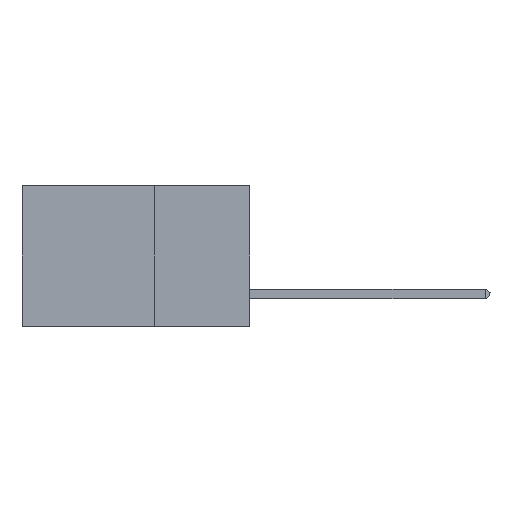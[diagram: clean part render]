
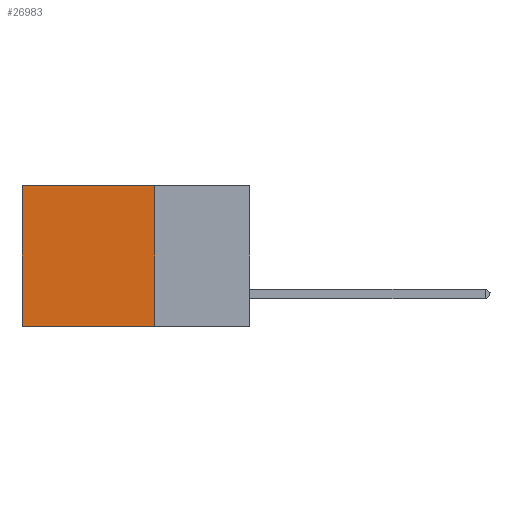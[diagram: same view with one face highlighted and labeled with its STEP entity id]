
A CAD part, left-side view. The second image highlights one B-rep face of the part: STEP entity #26983.
In plain terms, the highlighted planar face has unit normal (-1, 0, 0).
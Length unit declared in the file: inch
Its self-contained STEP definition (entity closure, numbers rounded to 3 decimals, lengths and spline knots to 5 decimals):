
#306 = VERTEX_POINT ( 'NONE', #31353 ) ;
#497 = VECTOR ( 'NONE', #8810, 39.37008 ) ;
#2908 = CARTESIAN_POINT ( 'NONE',  ( 0.2875, 0.25, 0. ) ) ;
#4172 = EDGE_CURVE ( 'NONE', #306, #19750, #36808, .T. ) ;
#5701 = CARTESIAN_POINT ( 'NONE',  ( 0.2875, 0.25, 0. ) ) ;
#5868 = PLANE ( 'NONE',  #14941 ) ;
#8810 = DIRECTION ( 'NONE',  ( 0., 1., 0. ) ) ;
#10869 = VECTOR ( 'NONE', #28611, 39.37008 ) ;
#12018 = ORIENTED_EDGE ( 'NONE', *, *, #26937, .T. ) ;
#12404 = CARTESIAN_POINT ( 'NONE',  ( 0.2875, 0.6, 0. ) ) ;
#13059 = DIRECTION ( 'NONE',  ( 1., 0., 0. ) ) ;
#13226 = CARTESIAN_POINT ( 'NONE',  ( 0.2875, 0.25, -0.37 ) ) ;
#13312 = DIRECTION ( 'NONE',  ( 0., 0., -1. ) ) ;
#13999 = FACE_OUTER_BOUND ( 'NONE', #15345, .T. ) ;
#14941 = AXIS2_PLACEMENT_3D ( 'NONE', #2908, #13059, #23271 ) ;
#15345 = EDGE_LOOP ( 'NONE', ( #32475, #23507, #39131, #12018 ) ) ;
#17144 = CARTESIAN_POINT ( 'NONE',  ( 0.2875, 0.25, 0. ) ) ;
#18142 = CARTESIAN_POINT ( 'NONE',  ( 0.2875, 0.6, -0.37 ) ) ;
#19750 = VERTEX_POINT ( 'NONE', #18142 ) ;
#20350 = VERTEX_POINT ( 'NONE', #33217 ) ;
#21724 = VECTOR ( 'NONE', #13312, 39.37008 ) ;
#22113 = LINE ( 'NONE', #5701, #497 ) ;
#22253 = LINE ( 'NONE', #17144, #24252 ) ;
#23271 = DIRECTION ( 'NONE',  ( 0., 0., -1. ) ) ;
#23507 = ORIENTED_EDGE ( 'NONE', *, *, #35232, .F. ) ;
#23815 = EDGE_CURVE ( 'NONE', #20350, #32720, #22253, .T. ) ;
#24252 = VECTOR ( 'NONE', #25397, 39.37008 ) ;
#25397 = DIRECTION ( 'NONE',  ( 0., 0., -1. ) ) ;
#26937 = EDGE_CURVE ( 'NONE', #20350, #306, #22113, .T. ) ;
#26983 = ADVANCED_FACE ( 'NONE', ( #13999 ), #5868, .F. ) ;
#27852 = CARTESIAN_POINT ( 'NONE',  ( 0.2875, 0.25, -0.37 ) ) ;
#28611 = DIRECTION ( 'NONE',  ( 0., 1., 0. ) ) ;
#31353 = CARTESIAN_POINT ( 'NONE',  ( 0.2875, 0.6, 0. ) ) ;
#32475 = ORIENTED_EDGE ( 'NONE', *, *, #4172, .T. ) ;
#32720 = VERTEX_POINT ( 'NONE', #27852 ) ;
#33217 = CARTESIAN_POINT ( 'NONE',  ( 0.2875, 0.25, 0. ) ) ;
#33302 = LINE ( 'NONE', #13226, #10869 ) ;
#35232 = EDGE_CURVE ( 'NONE', #32720, #19750, #33302, .T. ) ;
#36808 = LINE ( 'NONE', #12404, #21724 ) ;
#39131 = ORIENTED_EDGE ( 'NONE', *, *, #23815, .F. ) ;
